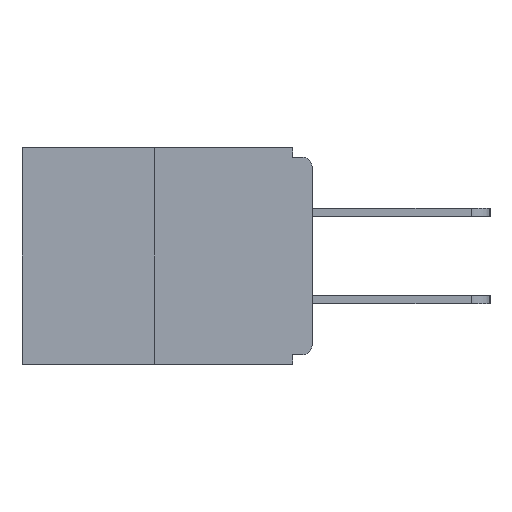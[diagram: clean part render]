
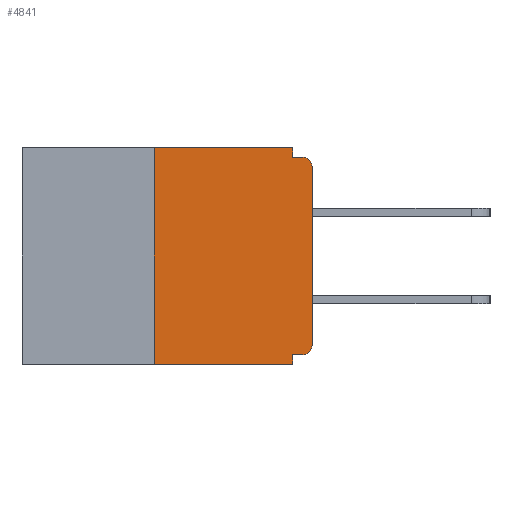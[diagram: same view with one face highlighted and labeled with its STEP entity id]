
A CAD part, left-side view. The second image highlights one B-rep face of the part: STEP entity #4841.
In plain terms, the highlighted planar face has unit normal (-1, 0, 0).
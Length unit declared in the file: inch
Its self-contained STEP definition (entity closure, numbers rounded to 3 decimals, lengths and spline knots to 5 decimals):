
#9 = LINE ( 'NONE', #8361, #1721 ) ;
#98 = DIRECTION ( 'NONE',  ( 0., 0., -1. ) ) ;
#204 = CARTESIAN_POINT ( 'NONE',  ( 0., 0.46, 0. ) ) ;
#1046 = DIRECTION ( 'NONE',  ( -1., 0., 0. ) ) ;
#1057 = AXIS2_PLACEMENT_3D ( 'NONE', #9435, #10512, #2496 ) ;
#1072 = ORIENTED_EDGE ( 'NONE', *, *, #14148, .F. ) ;
#1123 = CARTESIAN_POINT ( 'NONE',  ( 0., 0.015, -0.313 ) ) ;
#1148 = ORIENTED_EDGE ( 'NONE', *, *, #14889, .F. ) ;
#1468 = EDGE_CURVE ( 'NONE', #1892, #4169, #13935, .T. ) ;
#1509 = DIRECTION ( 'NONE',  ( 0., -1., 0. ) ) ;
#1616 = CARTESIAN_POINT ( 'NONE',  ( 0., 0.031, 0. ) ) ;
#1721 = VECTOR ( 'NONE', #12999, 39.37008 ) ;
#1763 = ORIENTED_EDGE ( 'NONE', *, *, #5616, .T. ) ;
#1892 = VERTEX_POINT ( 'NONE', #9208 ) ;
#1934 = VECTOR ( 'NONE', #12792, 39.37008 ) ;
#2176 = LINE ( 'NONE', #6572, #6534 ) ;
#2496 = DIRECTION ( 'NONE',  ( 0., 0., -1. ) ) ;
#2870 = VERTEX_POINT ( 'NONE', #11914 ) ;
#3117 = ORIENTED_EDGE ( 'NONE', *, *, #13088, .T. ) ;
#3153 = VERTEX_POINT ( 'NONE', #6853 ) ;
#3379 = DIRECTION ( 'NONE',  ( 0., 0., 1. ) ) ;
#3454 = ORIENTED_EDGE ( 'NONE', *, *, #8239, .F. ) ;
#3529 = CARTESIAN_POINT ( 'NONE',  ( 0., 0.031, 0. ) ) ;
#3544 = DIRECTION ( 'NONE',  ( 0., 0., -1. ) ) ;
#3575 = LINE ( 'NONE', #12852, #11467 ) ;
#3827 = CARTESIAN_POINT ( 'NONE',  ( 0., 0.46, 0. ) ) ;
#4060 = CARTESIAN_POINT ( 'NONE',  ( 0., 0., -0.328 ) ) ;
#4169 = VERTEX_POINT ( 'NONE', #9962 ) ;
#4174 = CARTESIAN_POINT ( 'NONE',  ( 0., 0.031, -0.328 ) ) ;
#4447 = VERTEX_POINT ( 'NONE', #4174 ) ;
#4659 = CARTESIAN_POINT ( 'NONE',  ( 0., 0.46, -0.343 ) ) ;
#4699 = ORIENTED_EDGE ( 'NONE', *, *, #10130, .F. ) ;
#4841 = ADVANCED_FACE ( 'NONE', ( #11981 ), #10779, .F. ) ;
#4907 = DIRECTION ( 'NONE',  ( 1., 0., 0. ) ) ;
#5228 = EDGE_CURVE ( 'NONE', #14444, #5749, #7948, .T. ) ;
#5469 = AXIS2_PLACEMENT_3D ( 'NONE', #204, #4907, #3544 ) ;
#5616 = EDGE_CURVE ( 'NONE', #10298, #2870, #9933, .T. ) ;
#5749 = VERTEX_POINT ( 'NONE', #7429 ) ;
#5753 = LINE ( 'NONE', #13942, #13822 ) ;
#5940 = DIRECTION ( 'NONE',  ( 0., 0., -1. ) ) ;
#6523 = LINE ( 'NONE', #4060, #9510 ) ;
#6534 = VECTOR ( 'NONE', #13595, 39.37008 ) ;
#6572 = CARTESIAN_POINT ( 'NONE',  ( 0., 0., -0.015 ) ) ;
#6853 = CARTESIAN_POINT ( 'NONE',  ( 0., 0.25, 0. ) ) ;
#7429 = CARTESIAN_POINT ( 'NONE',  ( 0., 0., -0.313 ) ) ;
#7622 = VERTEX_POINT ( 'NONE', #14717 ) ;
#7948 = CIRCLE ( 'NONE', #8695, 0.015 ) ;
#8113 = CARTESIAN_POINT ( 'NONE',  ( 0., 0., -0.03 ) ) ;
#8210 = ORIENTED_EDGE ( 'NONE', *, *, #1468, .T. ) ;
#8239 = EDGE_CURVE ( 'NONE', #4447, #4169, #3575, .T. ) ;
#8361 = CARTESIAN_POINT ( 'NONE',  ( 0., 0., 0. ) ) ;
#8515 = CARTESIAN_POINT ( 'NONE',  ( 0., 0.015, -0.328 ) ) ;
#8681 = VECTOR ( 'NONE', #1509, 39.37008 ) ;
#8695 = AXIS2_PLACEMENT_3D ( 'NONE', #1123, #1046, #98 ) ;
#9208 = CARTESIAN_POINT ( 'NONE',  ( 0., 0.25, -0.343 ) ) ;
#9261 = ORIENTED_EDGE ( 'NONE', *, *, #11051, .F. ) ;
#9435 = CARTESIAN_POINT ( 'NONE',  ( 0., 0.015, -0.03 ) ) ;
#9470 = EDGE_LOOP ( 'NONE', ( #15017, #9261, #8210, #3454, #1072, #13295, #3117, #1763, #4699, #1148 ) ) ;
#9510 = VECTOR ( 'NONE', #10078, 39.37008 ) ;
#9933 = CIRCLE ( 'NONE', #1057, 0.015 ) ;
#9962 = CARTESIAN_POINT ( 'NONE',  ( 0., 0.031, -0.343 ) ) ;
#10078 = DIRECTION ( 'NONE',  ( 0., 1., 0. ) ) ;
#10130 = EDGE_CURVE ( 'NONE', #7622, #2870, #2176, .T. ) ;
#10298 = VERTEX_POINT ( 'NONE', #8113 ) ;
#10512 = DIRECTION ( 'NONE',  ( -1., 0., 0. ) ) ;
#10779 = PLANE ( 'NONE',  #5469 ) ;
#10984 = LINE ( 'NONE', #3827, #8681 ) ;
#11051 = EDGE_CURVE ( 'NONE', #1892, #3153, #5753, .T. ) ;
#11181 = EDGE_CURVE ( 'NONE', #3153, #12251, #10984, .T. ) ;
#11467 = VECTOR ( 'NONE', #5940, 39.37008 ) ;
#11914 = CARTESIAN_POINT ( 'NONE',  ( 0., 0.015, -0.015 ) ) ;
#11981 = FACE_OUTER_BOUND ( 'NONE', #9470, .T. ) ;
#12209 = VECTOR ( 'NONE', #12298, 39.37008 ) ;
#12251 = VERTEX_POINT ( 'NONE', #3529 ) ;
#12298 = DIRECTION ( 'NONE',  ( 0., 0., -1. ) ) ;
#12792 = DIRECTION ( 'NONE',  ( 0., -1., 0. ) ) ;
#12852 = CARTESIAN_POINT ( 'NONE',  ( 0., 0.031, -0.343 ) ) ;
#12999 = DIRECTION ( 'NONE',  ( 0., 0., 1. ) ) ;
#13088 = EDGE_CURVE ( 'NONE', #5749, #10298, #9, .T. ) ;
#13295 = ORIENTED_EDGE ( 'NONE', *, *, #5228, .T. ) ;
#13566 = LINE ( 'NONE', #1616, #12209 ) ;
#13595 = DIRECTION ( 'NONE',  ( 0., -1., 0. ) ) ;
#13822 = VECTOR ( 'NONE', #3379, 39.37008 ) ;
#13935 = LINE ( 'NONE', #4659, #1934 ) ;
#13942 = CARTESIAN_POINT ( 'NONE',  ( 0., 0.25, 0. ) ) ;
#14148 = EDGE_CURVE ( 'NONE', #14444, #4447, #6523, .T. ) ;
#14444 = VERTEX_POINT ( 'NONE', #8515 ) ;
#14717 = CARTESIAN_POINT ( 'NONE',  ( 0., 0.031, -0.015 ) ) ;
#14889 = EDGE_CURVE ( 'NONE', #12251, #7622, #13566, .T. ) ;
#15017 = ORIENTED_EDGE ( 'NONE', *, *, #11181, .F. ) ;
